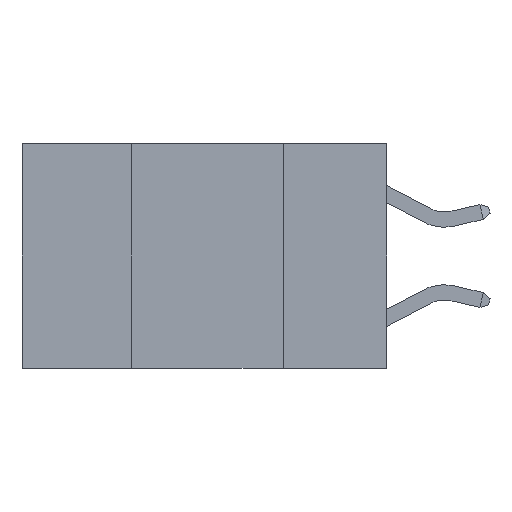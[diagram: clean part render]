
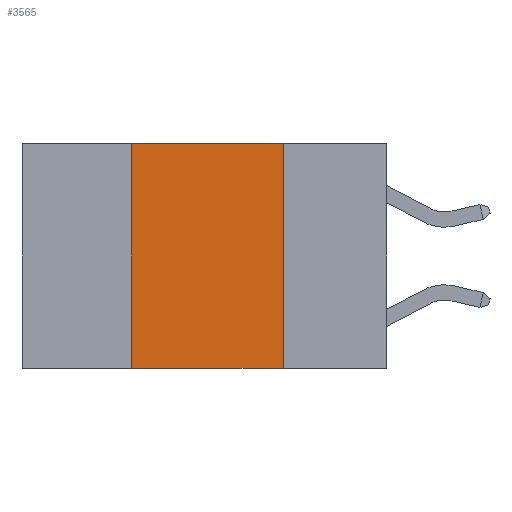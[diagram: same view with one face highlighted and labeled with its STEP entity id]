
A CAD part, left-side view. The second image highlights one B-rep face of the part: STEP entity #3565.
In plain terms, the highlighted planar face has unit normal (-1, 0, 0).
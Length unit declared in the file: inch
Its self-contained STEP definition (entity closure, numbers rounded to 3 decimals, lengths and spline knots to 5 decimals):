
#168 = CARTESIAN_POINT ( 'NONE',  ( 0., 0.17, -0.37 ) ) ;
#560 = CARTESIAN_POINT ( 'NONE',  ( 0., 0.17, 0. ) ) ;
#766 = VERTEX_POINT ( 'NONE', #7411 ) ;
#1279 = LINE ( 'NONE', #6739, #9419 ) ;
#1408 = DIRECTION ( 'NONE',  ( 0., 0., 1. ) ) ;
#1533 = CARTESIAN_POINT ( 'NONE',  ( 0., 0.42, 0. ) ) ;
#2239 = VECTOR ( 'NONE', #7726, 39.37008 ) ;
#2855 = ORIENTED_EDGE ( 'NONE', *, *, #9696, .F. ) ;
#3230 = DIRECTION ( 'NONE',  ( 0., 0., -1. ) ) ;
#3274 = DIRECTION ( 'NONE',  ( 0., -1., 0. ) ) ;
#3332 = VECTOR ( 'NONE', #1408, 39.37008 ) ;
#3565 = ADVANCED_FACE ( 'NONE', ( #9481 ), #4118, .F. ) ;
#4107 = DIRECTION ( 'NONE',  ( 0., -1., 0. ) ) ;
#4118 = PLANE ( 'NONE',  #8273 ) ;
#4170 = CARTESIAN_POINT ( 'NONE',  ( 0., 0.6, 0. ) ) ;
#4282 = VERTEX_POINT ( 'NONE', #168 ) ;
#4844 = EDGE_CURVE ( 'NONE', #5707, #8178, #5977, .T. ) ;
#4979 = CARTESIAN_POINT ( 'NONE',  ( 0., 0.6, 0. ) ) ;
#5292 = ORIENTED_EDGE ( 'NONE', *, *, #7998, .F. ) ;
#5325 = CARTESIAN_POINT ( 'NONE',  ( 0., 0.42, 0. ) ) ;
#5707 = VERTEX_POINT ( 'NONE', #7660 ) ;
#5977 = LINE ( 'NONE', #1533, #3332 ) ;
#5979 = EDGE_LOOP ( 'NONE', ( #2855, #5292, #8780, #8442 ) ) ;
#6617 = LINE ( 'NONE', #4170, #8043 ) ;
#6739 = CARTESIAN_POINT ( 'NONE',  ( 0., 0.6, -0.37 ) ) ;
#7411 = CARTESIAN_POINT ( 'NONE',  ( 0., 0.17, 0. ) ) ;
#7660 = CARTESIAN_POINT ( 'NONE',  ( 0., 0.42, -0.37 ) ) ;
#7667 = LINE ( 'NONE', #560, #2239 ) ;
#7726 = DIRECTION ( 'NONE',  ( 0., 0., -1. ) ) ;
#7998 = EDGE_CURVE ( 'NONE', #8178, #766, #6617, .T. ) ;
#8043 = VECTOR ( 'NONE', #4107, 39.37008 ) ;
#8178 = VERTEX_POINT ( 'NONE', #5325 ) ;
#8273 = AXIS2_PLACEMENT_3D ( 'NONE', #4979, #8516, #3230 ) ;
#8442 = ORIENTED_EDGE ( 'NONE', *, *, #9263, .T. ) ;
#8516 = DIRECTION ( 'NONE',  ( 1., 0., 0. ) ) ;
#8780 = ORIENTED_EDGE ( 'NONE', *, *, #4844, .F. ) ;
#9263 = EDGE_CURVE ( 'NONE', #5707, #4282, #1279, .T. ) ;
#9419 = VECTOR ( 'NONE', #3274, 39.37008 ) ;
#9481 = FACE_OUTER_BOUND ( 'NONE', #5979, .T. ) ;
#9696 = EDGE_CURVE ( 'NONE', #766, #4282, #7667, .T. ) ;
